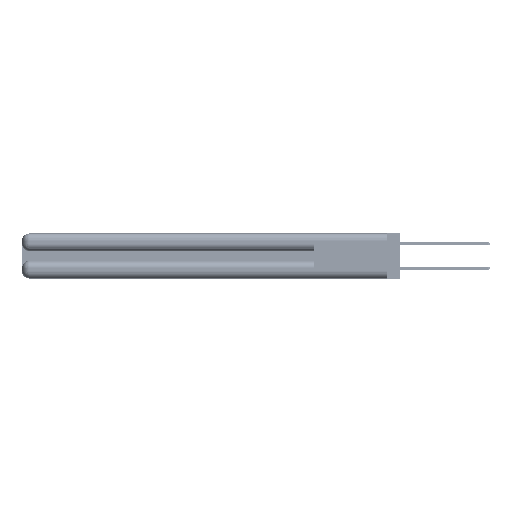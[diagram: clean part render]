
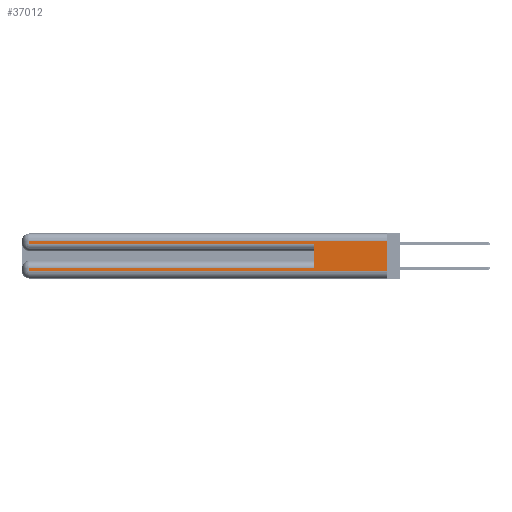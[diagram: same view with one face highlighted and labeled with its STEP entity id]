
A CAD part, left-side view. The second image highlights one B-rep face of the part: STEP entity #37012.
In plain terms, the highlighted planar face has unit normal (-1, 0, 0).
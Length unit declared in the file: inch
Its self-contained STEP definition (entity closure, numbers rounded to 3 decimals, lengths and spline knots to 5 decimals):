
#364 = VERTEX_POINT ( 'NONE', #46701 ) ;
#672 = DIRECTION ( 'NONE',  ( 0., 0., -1. ) ) ;
#2518 = EDGE_LOOP ( 'NONE', ( #40981, #19701, #34975, #52989, #5039, #30359, #20446, #13083 ) ) ;
#2657 = VERTEX_POINT ( 'NONE', #15061 ) ;
#3803 = CARTESIAN_POINT ( 'NONE',  ( 0., 2.94, 0.285 ) ) ;
#3992 = CARTESIAN_POINT ( 'NONE',  ( 0., 0., 0.06 ) ) ;
#5039 = ORIENTED_EDGE ( 'NONE', *, *, #13901, .F. ) ;
#7859 = CARTESIAN_POINT ( 'NONE',  ( 0., 2.94, 0.06 ) ) ;
#8046 = CARTESIAN_POINT ( 'NONE',  ( 0., 2.94, 0.37 ) ) ;
#9092 = CARTESIAN_POINT ( 'NONE',  ( 0., 2.94, 0.37 ) ) ;
#9935 = CARTESIAN_POINT ( 'NONE',  ( 0., 0., 0.285 ) ) ;
#10921 = LINE ( 'NONE', #15008, #32264 ) ;
#11102 = EDGE_CURVE ( 'NONE', #364, #34209, #17246, .T. ) ;
#11373 = VERTEX_POINT ( 'NONE', #7859 ) ;
#12062 = CARTESIAN_POINT ( 'NONE',  ( 0., 0., 0.37 ) ) ;
#13083 = ORIENTED_EDGE ( 'NONE', *, *, #13483, .T. ) ;
#13483 = EDGE_CURVE ( 'NONE', #11373, #2657, #19689, .T. ) ;
#13901 = EDGE_CURVE ( 'NONE', #50738, #43220, #10921, .T. ) ;
#14227 = EDGE_CURVE ( 'NONE', #50738, #19226, #51548, .T. ) ;
#14680 = FACE_OUTER_BOUND ( 'NONE', #2518, .T. ) ;
#15008 = CARTESIAN_POINT ( 'NONE',  ( 0., 0.6, 0.145 ) ) ;
#15061 = CARTESIAN_POINT ( 'NONE',  ( 0., 0., 0.06 ) ) ;
#16369 = DIRECTION ( 'NONE',  ( 1., 0., 0. ) ) ;
#16814 = CARTESIAN_POINT ( 'NONE',  ( 0., 2.94, 0.085 ) ) ;
#17246 = LINE ( 'NONE', #52592, #48488 ) ;
#18238 = EDGE_CURVE ( 'NONE', #23496, #43220, #34514, .T. ) ;
#19200 = CARTESIAN_POINT ( 'NONE',  ( 0., 0., 0.37 ) ) ;
#19226 = VERTEX_POINT ( 'NONE', #16814 ) ;
#19243 = CARTESIAN_POINT ( 'NONE',  ( 0., 2.94, 0.31 ) ) ;
#19689 = LINE ( 'NONE', #3992, #29591 ) ;
#19701 = ORIENTED_EDGE ( 'NONE', *, *, #11102, .T. ) ;
#20446 = ORIENTED_EDGE ( 'NONE', *, *, #53434, .T. ) ;
#21889 = CARTESIAN_POINT ( 'NONE',  ( 0., 0., 0.085 ) ) ;
#23496 = VERTEX_POINT ( 'NONE', #3803 ) ;
#23499 = CARTESIAN_POINT ( 'NONE',  ( 0., 0.6, 0.285 ) ) ;
#23535 = DIRECTION ( 'NONE',  ( 0., 0., 1. ) ) ;
#24525 = VECTOR ( 'NONE', #39765, 39.37008 ) ;
#25197 = DIRECTION ( 'NONE',  ( 0., 0., -1. ) ) ;
#25349 = LINE ( 'NONE', #19200, #45318 ) ;
#26102 = DIRECTION ( 'NONE',  ( 0., 1., 0. ) ) ;
#26431 = AXIS2_PLACEMENT_3D ( 'NONE', #12062, #16369, #46124 ) ;
#27524 = VECTOR ( 'NONE', #26102, 39.37008 ) ;
#28334 = VECTOR ( 'NONE', #25197, 39.37008 ) ;
#29591 = VECTOR ( 'NONE', #46477, 39.37008 ) ;
#29666 = LINE ( 'NONE', #8046, #28334 ) ;
#30359 = ORIENTED_EDGE ( 'NONE', *, *, #14227, .T. ) ;
#32264 = VECTOR ( 'NONE', #23535, 39.37008 ) ;
#33577 = CARTESIAN_POINT ( 'NONE',  ( 0., 0.6, 0.085 ) ) ;
#34209 = VERTEX_POINT ( 'NONE', #19243 ) ;
#34514 = LINE ( 'NONE', #9935, #24525 ) ;
#34975 = ORIENTED_EDGE ( 'NONE', *, *, #40714, .T. ) ;
#36274 = DIRECTION ( 'NONE',  ( 0., 0., -1. ) ) ;
#36801 = EDGE_CURVE ( 'NONE', #364, #2657, #25349, .T. ) ;
#37012 = ADVANCED_FACE ( 'NONE', ( #14680 ), #37568, .F. ) ;
#37568 = PLANE ( 'NONE',  #26431 ) ;
#39765 = DIRECTION ( 'NONE',  ( 0., -1., 0. ) ) ;
#39932 = DIRECTION ( 'NONE',  ( 0., 1., 0. ) ) ;
#40714 = EDGE_CURVE ( 'NONE', #34209, #23496, #29666, .T. ) ;
#40981 = ORIENTED_EDGE ( 'NONE', *, *, #36801, .F. ) ;
#43220 = VERTEX_POINT ( 'NONE', #23499 ) ;
#45318 = VECTOR ( 'NONE', #36274, 39.37008 ) ;
#46124 = DIRECTION ( 'NONE',  ( 0., 0., -1. ) ) ;
#46477 = DIRECTION ( 'NONE',  ( 0., -1., 0. ) ) ;
#46701 = CARTESIAN_POINT ( 'NONE',  ( 0., 0., 0.31 ) ) ;
#48488 = VECTOR ( 'NONE', #39932, 39.37008 ) ;
#50738 = VERTEX_POINT ( 'NONE', #33577 ) ;
#50925 = VECTOR ( 'NONE', #672, 39.37008 ) ;
#51548 = LINE ( 'NONE', #21889, #27524 ) ;
#52258 = LINE ( 'NONE', #9092, #50925 ) ;
#52592 = CARTESIAN_POINT ( 'NONE',  ( 0., 0., 0.31 ) ) ;
#52989 = ORIENTED_EDGE ( 'NONE', *, *, #18238, .T. ) ;
#53434 = EDGE_CURVE ( 'NONE', #19226, #11373, #52258, .T. ) ;
